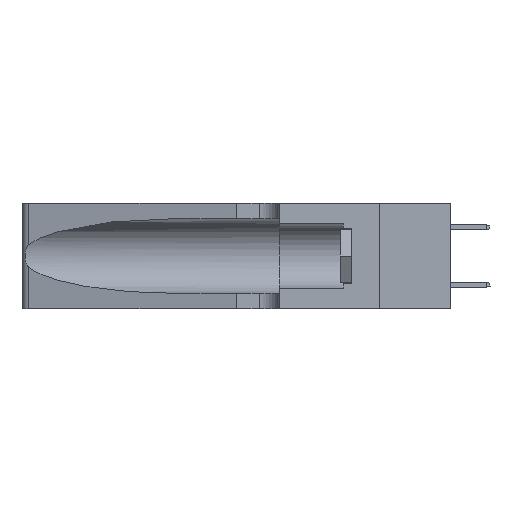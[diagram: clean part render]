
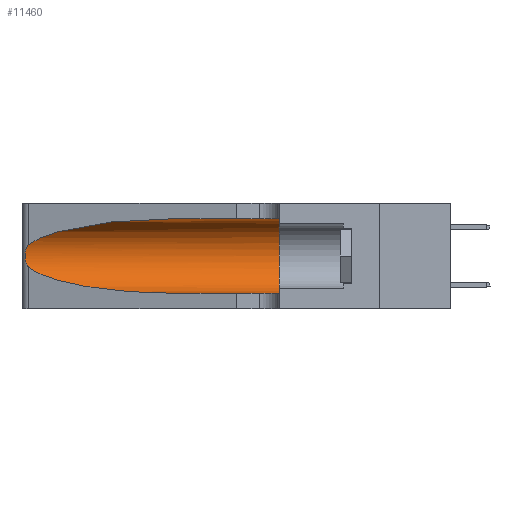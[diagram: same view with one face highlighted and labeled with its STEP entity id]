
A CAD part, left-side view. The second image highlights one B-rep face of the part: STEP entity #11460.
In plain terms, the highlighted cylindrical face has radius 3.308 mm (diameter 6.617 mm), a partial arc.
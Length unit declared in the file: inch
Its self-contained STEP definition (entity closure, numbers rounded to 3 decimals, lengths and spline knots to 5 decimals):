
#525 = DIRECTION ( 'NONE',  ( 0., -1., 0. ) ) ;
#529 = CYLINDRICAL_SURFACE ( 'NONE', #6479, 0.13025 ) ;
#981 = VERTEX_POINT ( 'NONE', #19636 ) ;
#1101 = CARTESIAN_POINT ( 'NONE',  ( 0.25487, 1.22718, 0.22369 ) ) ;
#1601 = CARTESIAN_POINT ( 'NONE',  ( 0.18966, 0.96281, 0.31525 ) ) ;
#1744 = CARTESIAN_POINT ( 'NONE',  ( 0.1305, 0.72297, 0.05475 ) ) ;
#2103 = DIRECTION ( 'NONE',  ( 0., 0., -1. ) ) ;
#2978 = CARTESIAN_POINT ( 'NONE',  ( 0.25787, 1.23484, 0.2124 ) ) ;
#3068 = CARTESIAN_POINT ( 'NONE',  ( 0.25487, 1.22718, 0.22369 ) ) ;
#3196 = CARTESIAN_POINT ( 'NONE',  ( 0.2373, 1.15595, 0.08982 ) ) ;
#3686 = FACE_OUTER_BOUND ( 'NONE', #20307, .T. ) ;
#3777 = VERTEX_POINT ( 'NONE', #9165 ) ;
#3779 = LINE ( 'NONE', #10432, #13770 ) ;
#3783 = DIRECTION ( 'NONE',  ( 0., -1., 0. ) ) ;
#4349 = CARTESIAN_POINT ( 'NONE',  ( 0.26018, 1.23835, 0.19895 ) ) ;
#4565 = CARTESIAN_POINT ( 'NONE',  ( 0.26075, 1.23896, 0.178 ) ) ;
#4566 = VERTEX_POINT ( 'NONE', #6489 ) ;
#6082 = DIRECTION ( 'NONE',  ( 0., -1., 0. ) ) ;
#6234 = EDGE_CURVE ( 'NONE', #16901, #6954, #3779, .T. ) ;
#6248 = CARTESIAN_POINT ( 'NONE',  ( 0.1305, 0.72297, 0.05475 ) ) ;
#6479 = AXIS2_PLACEMENT_3D ( 'NONE', #16612, #3783, #2103 ) ;
#6489 = CARTESIAN_POINT ( 'NONE',  ( 0.1305, 0.72297, 0.31525 ) ) ;
#6879 = EDGE_CURVE ( 'NONE', #14242, #16901, #15901, .T. ) ;
#6954 = VERTEX_POINT ( 'NONE', #8602 ) ;
#7379 =( BOUNDED_CURVE ( )  B_SPLINE_CURVE ( 3, ( #20766, #1601, #11095, #3068 ),
 .UNSPECIFIED., .F., .F. ) 
 B_SPLINE_CURVE_WITH_KNOTS ( ( 4, 4 ),
 ( 1.5708, 2.84003 ),
 .UNSPECIFIED. ) 
 CURVE ( )  GEOMETRIC_REPRESENTATION_ITEM ( )  RATIONAL_B_SPLINE_CURVE ( ( 1., 0.87, 0.87, 1. ) ) 
 REPRESENTATION_ITEM ( '' )  );
#7547 = CARTESIAN_POINT ( 'NONE',  ( 0.26017, 1.23833, 0.17102 ) ) ;
#7646 = CARTESIAN_POINT ( 'NONE',  ( 0.25639, 1.23184, 0.21858 ) ) ;
#7740 = ORIENTED_EDGE ( 'NONE', *, *, #6234, .T. ) ;
#7977 = CIRCLE ( 'NONE', #16090, 0.13025 ) ;
#8602 = CARTESIAN_POINT ( 'NONE',  ( 0.1305, 0.35, 0.05475 ) ) ;
#9152 = DIRECTION ( 'NONE',  ( 0., 1., 0. ) ) ;
#9165 = CARTESIAN_POINT ( 'NONE',  ( 0.25487, 1.22718, 0.22369 ) ) ;
#9228 = CARTESIAN_POINT ( 'NONE',  ( 0.25487, 1.22718, 0.14631 ) ) ;
#9434 = CARTESIAN_POINT ( 'NONE',  ( 0.25856, 1.23593, 0.16098 ) ) ;
#9527 = EDGE_CURVE ( 'NONE', #4566, #981, #14100, .T. ) ;
#10432 = CARTESIAN_POINT ( 'NONE',  ( 0.1305, 1.61858, 0.05475 ) ) ;
#10628 = ORIENTED_EDGE ( 'NONE', *, *, #6879, .T. ) ;
#10805 = CARTESIAN_POINT ( 'NONE',  ( 0.25555, 1.22994, 0.2215 ) ) ;
#11095 = CARTESIAN_POINT ( 'NONE',  ( 0.2373, 1.15595, 0.28018 ) ) ;
#11288 = ORIENTED_EDGE ( 'NONE', *, *, #9527, .F. ) ;
#11460 = ADVANCED_FACE ( 'NONE', ( #3686 ), #529, .F. ) ;
#12231 = CARTESIAN_POINT ( 'NONE',  ( 0.1305, 0.35, 0.185 ) ) ;
#12234 = EDGE_CURVE ( 'NONE', #4566, #3777, #7379, .T. ) ;
#12515 = CARTESIAN_POINT ( 'NONE',  ( 0.25789, 1.23486, 0.15765 ) ) ;
#13770 = VECTOR ( 'NONE', #525, 39.37008 ) ;
#14097 = ORIENTED_EDGE ( 'NONE', *, *, #20610, .T. ) ;
#14100 = LINE ( 'NONE', #20396, #15530 ) ;
#14186 = CARTESIAN_POINT ( 'NONE',  ( 0.26075, 1.23896, 0.19203 ) ) ;
#14242 = VERTEX_POINT ( 'NONE', #16772 ) ;
#15489 = CARTESIAN_POINT ( 'NONE',  ( 0.25854, 1.2359, 0.20912 ) ) ;
#15530 = VECTOR ( 'NONE', #6082, 39.37008 ) ;
#15901 =( BOUNDED_CURVE ( )  B_SPLINE_CURVE ( 3, ( #17729, #3196, #17834, #1744 ),
 .UNSPECIFIED., .F., .F. ) 
 B_SPLINE_CURVE_WITH_KNOTS ( ( 4, 4 ),
 ( 3.44316, 4.71239 ),
 .UNSPECIFIED. ) 
 CURVE ( )  GEOMETRIC_REPRESENTATION_ITEM ( )  RATIONAL_B_SPLINE_CURVE ( ( 1., 0.87, 0.87, 1. ) ) 
 REPRESENTATION_ITEM ( '' )  );
#15907 = CARTESIAN_POINT ( 'NONE',  ( 0.25639, 1.23186, 0.15144 ) ) ;
#16090 = AXIS2_PLACEMENT_3D ( 'NONE', #12231, #9152, #20492 ) ;
#16612 = CARTESIAN_POINT ( 'NONE',  ( 0.1305, 1.61858, 0.185 ) ) ;
#16772 = CARTESIAN_POINT ( 'NONE',  ( 0.25487, 1.22718, 0.14631 ) ) ;
#16901 = VERTEX_POINT ( 'NONE', #6248 ) ;
#17292 = CARTESIAN_POINT ( 'NONE',  ( 0.25555, 1.22993, 0.14849 ) ) ;
#17729 = CARTESIAN_POINT ( 'NONE',  ( 0.25487, 1.22718, 0.14631 ) ) ;
#17834 = CARTESIAN_POINT ( 'NONE',  ( 0.18966, 0.96281, 0.05475 ) ) ;
#18341 = ORIENTED_EDGE ( 'NONE', *, *, #12234, .T. ) ;
#18387 = B_SPLINE_CURVE_WITH_KNOTS ( 'NONE', 3,
 ( #1101, #10805, #7646, #2978, #15489, #4349, #14186, #4565, #7547, #9434, #12515, #15907, #17292, #9228 ),
 .UNSPECIFIED., .F., .F.,
 ( 4, 2, 2, 2, 2, 2, 4 ),
 ( 0., 0.00027, 0.00053, 0.00107, 0.0016, 0.00187, 0.00214 ),
 .UNSPECIFIED. ) ;
#18820 = EDGE_CURVE ( 'NONE', #981, #6954, #7977, .T. ) ;
#19636 = CARTESIAN_POINT ( 'NONE',  ( 0.1305, 0.35, 0.31525 ) ) ;
#20071 = ORIENTED_EDGE ( 'NONE', *, *, #18820, .F. ) ;
#20307 = EDGE_LOOP ( 'NONE', ( #18341, #14097, #10628, #7740, #20071, #11288 ) ) ;
#20396 = CARTESIAN_POINT ( 'NONE',  ( 0.1305, 1.61858, 0.31525 ) ) ;
#20492 = DIRECTION ( 'NONE',  ( 0., 0., 1. ) ) ;
#20610 = EDGE_CURVE ( 'NONE', #3777, #14242, #18387, .T. ) ;
#20766 = CARTESIAN_POINT ( 'NONE',  ( 0.1305, 0.72297, 0.31525 ) ) ;
